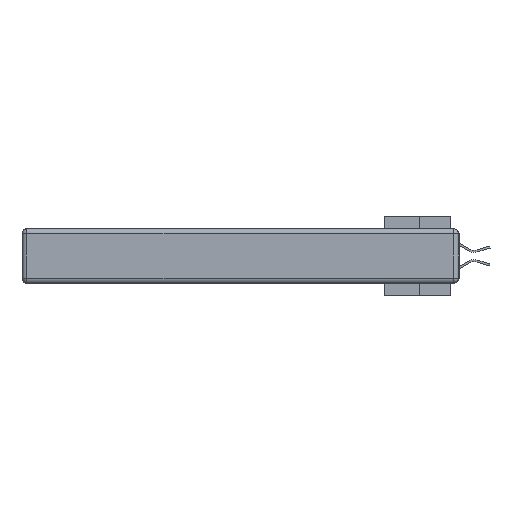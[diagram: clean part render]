
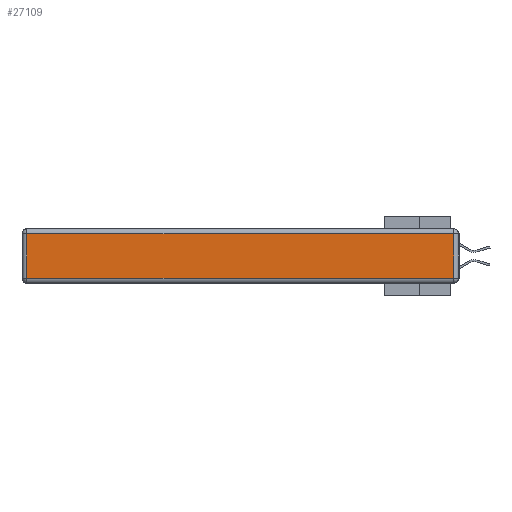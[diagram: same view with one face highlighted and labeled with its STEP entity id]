
A CAD part, left-side view. The second image highlights one B-rep face of the part: STEP entity #27109.
In plain terms, the highlighted planar face has unit normal (-1, 0, 0).
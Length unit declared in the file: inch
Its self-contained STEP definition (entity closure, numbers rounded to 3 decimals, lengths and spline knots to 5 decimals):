
#67 = DIRECTION ( 'NONE',  ( 0., 0., 1. ) ) ;
#306 = VECTOR ( 'NONE', #21988, 39.37008 ) ;
#2243 = VECTOR ( 'NONE', #31165, 39.37008 ) ;
#2759 = CARTESIAN_POINT ( 'NONE',  ( 0., 0., -0.343 ) ) ;
#2871 = VERTEX_POINT ( 'NONE', #10673 ) ;
#2924 = DIRECTION ( 'NONE',  ( 0., 0., -1. ) ) ;
#4192 = ORIENTED_EDGE ( 'NONE', *, *, #15057, .T. ) ;
#4858 = ORIENTED_EDGE ( 'NONE', *, *, #26811, .T. ) ;
#6475 = LINE ( 'NONE', #8106, #30916 ) ;
#8102 = LINE ( 'NONE', #8964, #29581 ) ;
#8106 = CARTESIAN_POINT ( 'NONE',  ( 0., 2.72, -0.343 ) ) ;
#8465 = CARTESIAN_POINT ( 'NONE',  ( 0., 0., -0.313 ) ) ;
#8937 = LINE ( 'NONE', #28355, #2243 ) ;
#8964 = CARTESIAN_POINT ( 'NONE',  ( 0., 0.03, -0.343 ) ) ;
#9982 = VERTEX_POINT ( 'NONE', #33272 ) ;
#10673 = CARTESIAN_POINT ( 'NONE',  ( 0., 0.03, -0.313 ) ) ;
#11330 = EDGE_LOOP ( 'NONE', ( #14662, #4192, #4858, #32293 ) ) ;
#11906 = EDGE_CURVE ( 'NONE', #12658, #2871, #24695, .T. ) ;
#12414 = CARTESIAN_POINT ( 'NONE',  ( 0., 2.72, -0.313 ) ) ;
#12658 = VERTEX_POINT ( 'NONE', #12414 ) ;
#13129 = FACE_OUTER_BOUND ( 'NONE', #11330, .T. ) ;
#13757 = VERTEX_POINT ( 'NONE', #27914 ) ;
#14662 = ORIENTED_EDGE ( 'NONE', *, *, #11906, .T. ) ;
#15057 = EDGE_CURVE ( 'NONE', #2871, #9982, #8102, .T. ) ;
#18630 = PLANE ( 'NONE',  #23994 ) ;
#21988 = DIRECTION ( 'NONE',  ( 0., -1., 0. ) ) ;
#23994 = AXIS2_PLACEMENT_3D ( 'NONE', #2759, #29510, #67 ) ;
#24695 = LINE ( 'NONE', #8465, #306 ) ;
#26811 = EDGE_CURVE ( 'NONE', #9982, #13757, #8937, .T. ) ;
#27109 = ADVANCED_FACE ( 'NONE', ( #13129 ), #18630, .T. ) ;
#27914 = CARTESIAN_POINT ( 'NONE',  ( 0., 2.72, -0.03 ) ) ;
#28286 = EDGE_CURVE ( 'NONE', #13757, #12658, #6475, .T. ) ;
#28355 = CARTESIAN_POINT ( 'NONE',  ( 0., 2.75, -0.03 ) ) ;
#29510 = DIRECTION ( 'NONE',  ( -1., 0., 0. ) ) ;
#29581 = VECTOR ( 'NONE', #33102, 39.37008 ) ;
#30916 = VECTOR ( 'NONE', #2924, 39.37008 ) ;
#31165 = DIRECTION ( 'NONE',  ( 0., 1., 0. ) ) ;
#32293 = ORIENTED_EDGE ( 'NONE', *, *, #28286, .T. ) ;
#33102 = DIRECTION ( 'NONE',  ( 0., 0., 1. ) ) ;
#33272 = CARTESIAN_POINT ( 'NONE',  ( 0., 0.03, -0.03 ) ) ;
